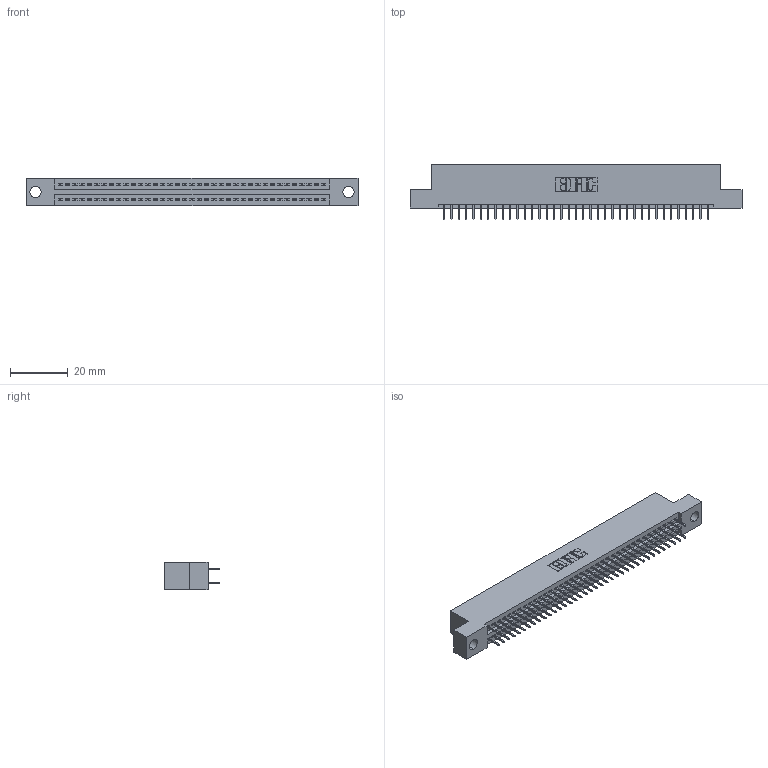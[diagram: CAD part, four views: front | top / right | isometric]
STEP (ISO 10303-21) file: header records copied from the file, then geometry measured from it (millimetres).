
FILE_DESCRIPTION (( 'STEP AP203' ), '1' );
FILE_NAME ('395-074-524-204.STEP', '2021-06-17T05:25:40', ( '' ), ( '' ), 'SwSTEP 2.0', 'SolidWorks 2020', '' );
FILE_SCHEMA (( 'CONFIG_CONTROL_DESIGN' ));
Length unit declared in the file: inch
Products named in the file (3): 395-074-524-204; 345-292-001_345-293-124; 345 Part_Flush Mounting Lugs - 0.156 Dia-TI
Assembly tree (75 placements, depth 2):
  395-074-524-204
    345 Part_Flush Mounting Lugs - 0.156 Dia-TI
    345-292-001_345-293-124  x74
Bounding box: 115.19 x 19.35 x 9.4 mm (x, y, z)
Volume: 10925.2 mm3; surface area: 15608.5 mm2
Topology: 75 solids, 75 shells, 4136 faces, 11699 edges, 7502 vertices
Faces by surface type: plane 2980, cylinder 1156
Entity records: 30197 total; most frequent: CARTESIAN_POINT 5070, ORIENTED_EDGE 5002, DIRECTION 4477, EDGE_CURVE 2501, LINE 2225, VECTOR 2225, VERTEX_POINT 1662, AXIS2_PLACEMENT_3D 1126
